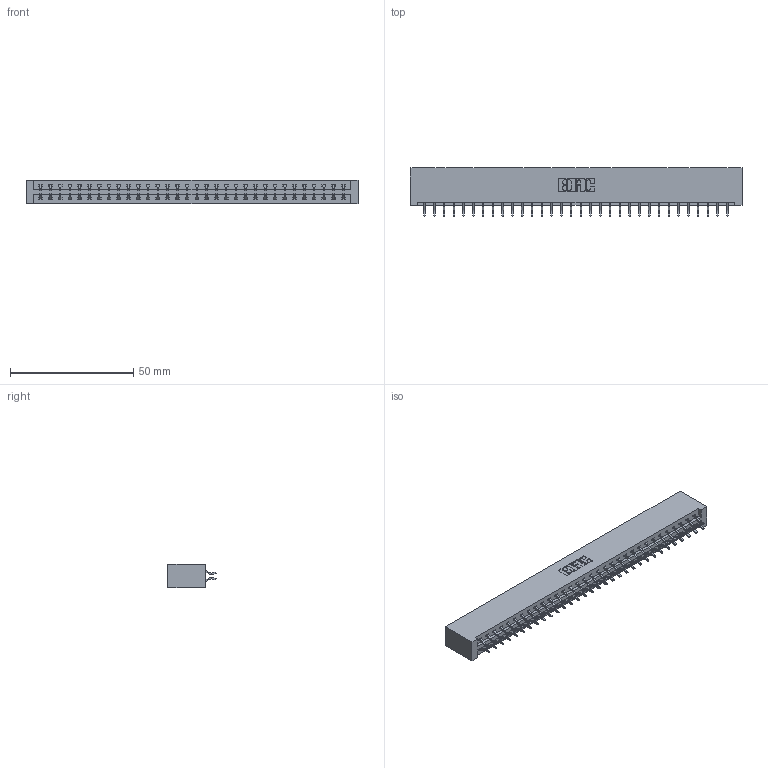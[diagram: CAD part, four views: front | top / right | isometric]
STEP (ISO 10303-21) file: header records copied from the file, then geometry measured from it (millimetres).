
FILE_DESCRIPTION (( 'STEP AP203' ), '1' );
FILE_NAME ('337-064-556-201.STEP', '2018-08-11T06:30:26', ( '' ), ( '' ), 'SwSTEP 2.0', 'SolidWorks 2016', '' );
FILE_SCHEMA (( 'CONFIG_CONTROL_DESIGN' ));
Length unit declared in the file: inch
Products named in the file (3): 337 Part_No Mounting Lugs; 345-292-001_556 Tail; 337-064-556-201
Assembly tree (65 placements, depth 2):
  337-064-556-201
    337 Part_No Mounting Lugs
    345-292-001_556 Tail  x64
Bounding box: 134.67 x 19.57 x 9.4 mm (x, y, z)
Volume: 14817.8 mm3; surface area: 16643 mm2
Topology: 65 solids, 65 shells, 3946 faces, 11743 edges, 7742 vertices
Faces by surface type: plane 2754, cylinder 1192
Entity records: 26047 total; most frequent: CARTESIAN_POINT 4410, ORIENTED_EDGE 4334, DIRECTION 3751, EDGE_CURVE 2167, VECTOR 2039, LINE 2039, VERTEX_POINT 1442, AXIS2_PLACEMENT_3D 856
